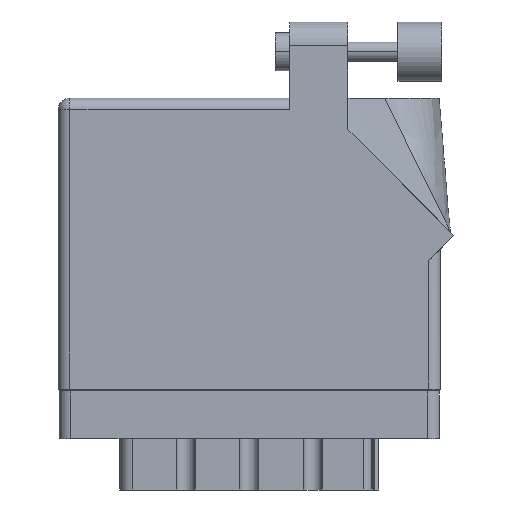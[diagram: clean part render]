
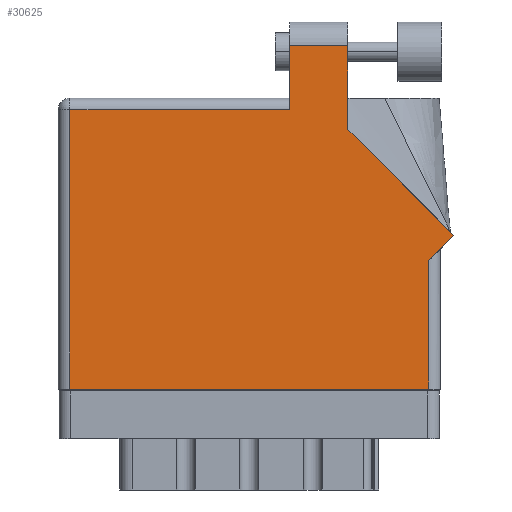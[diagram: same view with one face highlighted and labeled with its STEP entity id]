
A CAD part, front view. The second image highlights one B-rep face of the part: STEP entity #30625.
In plain terms, the highlighted face is planar.
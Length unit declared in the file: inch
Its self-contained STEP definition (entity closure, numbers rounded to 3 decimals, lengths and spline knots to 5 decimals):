
#703 = DIRECTION ( 'NONE',  ( 0., -1., 0. ) ) ;
#728 = PLANE ( 'NONE',  #29909 ) ;
#1012 = VECTOR ( 'NONE', #27069, 39.37008 ) ;
#1538 = CARTESIAN_POINT ( 'NONE',  ( 1.217, 1.805, 0. ) ) ;
#3522 = DIRECTION ( 'NONE',  ( -1., 0., 0. ) ) ;
#3683 = DIRECTION ( 'NONE',  ( -1., 0., 0. ) ) ;
#3808 = CARTESIAN_POINT ( 'NONE',  ( 1.524, 1.36442, 0. ) ) ;
#4062 = ORIENTED_EDGE ( 'NONE', *, *, #30048, .T. ) ;
#4425 = DIRECTION ( 'NONE',  ( -1., 0., 0. ) ) ;
#6077 = LINE ( 'NONE', #14223, #15100 ) ;
#6141 = VERTEX_POINT ( 'NONE', #19053 ) ;
#6703 = FACE_OUTER_BOUND ( 'NONE', #15080, .T. ) ;
#7651 = VERTEX_POINT ( 'NONE', #18878 ) ;
#7905 = CARTESIAN_POINT ( 'NONE',  ( 1.948, 0., 0. ) ) ;
#8319 = CARTESIAN_POINT ( 'NONE',  ( 1.217, 1.805, 0. ) ) ;
#8336 = LINE ( 'NONE', #21283, #32518 ) ;
#8933 = VERTEX_POINT ( 'NONE', #16599 ) ;
#9724 = DIRECTION ( 'NONE',  ( 0., 1., 0. ) ) ;
#10430 = ORIENTED_EDGE ( 'NONE', *, *, #28399, .T. ) ;
#10454 = EDGE_CURVE ( 'NONE', #34608, #34826, #21380, .T. ) ;
#10707 = VECTOR ( 'NONE', #24193, 39.37008 ) ;
#14121 = ORIENTED_EDGE ( 'NONE', *, *, #22616, .T. ) ;
#14223 = CARTESIAN_POINT ( 'NONE',  ( 1.217, 1.53, 0. ) ) ;
#14458 = ORIENTED_EDGE ( 'NONE', *, *, #36663, .T. ) ;
#15080 = EDGE_LOOP ( 'NONE', ( #21940, #14121, #36771, #4062, #14458, #33918, #23702, #10430, #22905 ) ) ;
#15100 = VECTOR ( 'NONE', #36858, 39.37008 ) ;
#16377 = DIRECTION ( 'NONE',  ( 0., 1., 0. ) ) ;
#16599 = CARTESIAN_POINT ( 'NONE',  ( 1.217, 1.468, 0. ) ) ;
#16669 = EDGE_CURVE ( 'NONE', #34858, #34608, #35812, .T. ) ;
#17612 = LINE ( 'NONE', #30436, #27489 ) ;
#18878 = CARTESIAN_POINT ( 'NONE',  ( 0.062, 1.468, 0. ) ) ;
#19053 = CARTESIAN_POINT ( 'NONE',  ( 1.524, 1.805, 0. ) ) ;
#20618 = DIRECTION ( 'NONE',  ( 0., 0., -1. ) ) ;
#20838 = CARTESIAN_POINT ( 'NONE',  ( 1.948, 0.675, 0. ) ) ;
#21283 = CARTESIAN_POINT ( 'NONE',  ( 1.524, 1.36442, 0. ) ) ;
#21380 = LINE ( 'NONE', #33738, #36115 ) ;
#21938 = DIRECTION ( 'NONE',  ( -0.707, 0.707, 0. ) ) ;
#21940 = ORIENTED_EDGE ( 'NONE', *, *, #26296, .T. ) ;
#22141 = LINE ( 'NONE', #24189, #1012 ) ;
#22458 = VERTEX_POINT ( 'NONE', #3808 ) ;
#22616 = EDGE_CURVE ( 'NONE', #6141, #35663, #34922, .T. ) ;
#22905 = ORIENTED_EDGE ( 'NONE', *, *, #35142, .T. ) ;
#23195 = CARTESIAN_POINT ( 'NONE',  ( 0.062, 0., 0. ) ) ;
#23702 = ORIENTED_EDGE ( 'NONE', *, *, #10454, .T. ) ;
#24189 = CARTESIAN_POINT ( 'NONE',  ( 2.01, 0.737, 0. ) ) ;
#24193 = DIRECTION ( 'NONE',  ( 1., 0., 0. ) ) ;
#25799 = VERTEX_POINT ( 'NONE', #33419 ) ;
#26296 = EDGE_CURVE ( 'NONE', #22458, #6141, #8336, .T. ) ;
#27069 = DIRECTION ( 'NONE',  ( 0.707, 0.707, 0. ) ) ;
#27306 = VECTOR ( 'NONE', #4425, 39.37008 ) ;
#27348 = LINE ( 'NONE', #29073, #34964 ) ;
#27489 = VECTOR ( 'NONE', #21938, 39.37008 ) ;
#28399 = EDGE_CURVE ( 'NONE', #34826, #25799, #22141, .T. ) ;
#29073 = CARTESIAN_POINT ( 'NONE',  ( 0.062, 0., 0. ) ) ;
#29639 = LINE ( 'NONE', #35644, #35925 ) ;
#29909 = AXIS2_PLACEMENT_3D ( 'NONE', #34990, #20618, #3522 ) ;
#30048 = EDGE_CURVE ( 'NONE', #8933, #7651, #29639, .T. ) ;
#30436 = CARTESIAN_POINT ( 'NONE',  ( 2.08071, 0.80771, 0. ) ) ;
#30625 = ADVANCED_FACE ( 'NONE', ( #6703 ), #728, .F. ) ;
#32192 = CARTESIAN_POINT ( 'NONE',  ( 0., 0., 0. ) ) ;
#32518 = VECTOR ( 'NONE', #9724, 39.37008 ) ;
#33021 = EDGE_CURVE ( 'NONE', #35663, #8933, #6077, .T. ) ;
#33419 = CARTESIAN_POINT ( 'NONE',  ( 2.08071, 0.80771, 0. ) ) ;
#33738 = CARTESIAN_POINT ( 'NONE',  ( 1.948, 0.737, 0. ) ) ;
#33918 = ORIENTED_EDGE ( 'NONE', *, *, #16669, .T. ) ;
#34608 = VERTEX_POINT ( 'NONE', #7905 ) ;
#34826 = VERTEX_POINT ( 'NONE', #20838 ) ;
#34858 = VERTEX_POINT ( 'NONE', #23195 ) ;
#34922 = LINE ( 'NONE', #8319, #27306 ) ;
#34964 = VECTOR ( 'NONE', #703, 39.37008 ) ;
#34990 = CARTESIAN_POINT ( 'NONE',  ( 0., 1.53, 0. ) ) ;
#35142 = EDGE_CURVE ( 'NONE', #25799, #22458, #17612, .T. ) ;
#35644 = CARTESIAN_POINT ( 'NONE',  ( 0., 1.468, 0. ) ) ;
#35663 = VERTEX_POINT ( 'NONE', #1538 ) ;
#35812 = LINE ( 'NONE', #32192, #10707 ) ;
#35925 = VECTOR ( 'NONE', #3683, 39.37008 ) ;
#36115 = VECTOR ( 'NONE', #16377, 39.37008 ) ;
#36663 = EDGE_CURVE ( 'NONE', #7651, #34858, #27348, .T. ) ;
#36771 = ORIENTED_EDGE ( 'NONE', *, *, #33021, .T. ) ;
#36858 = DIRECTION ( 'NONE',  ( 0., -1., 0. ) ) ;
